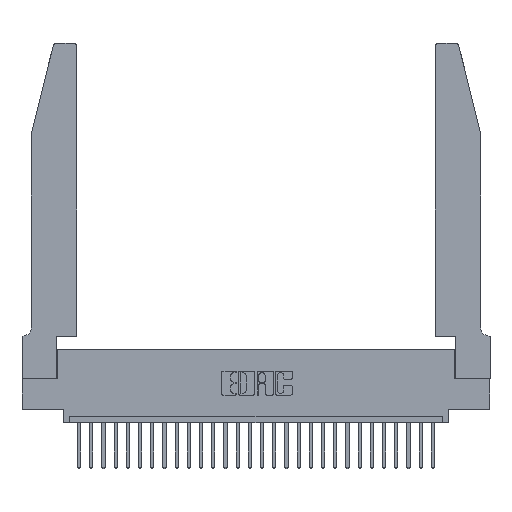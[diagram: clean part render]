
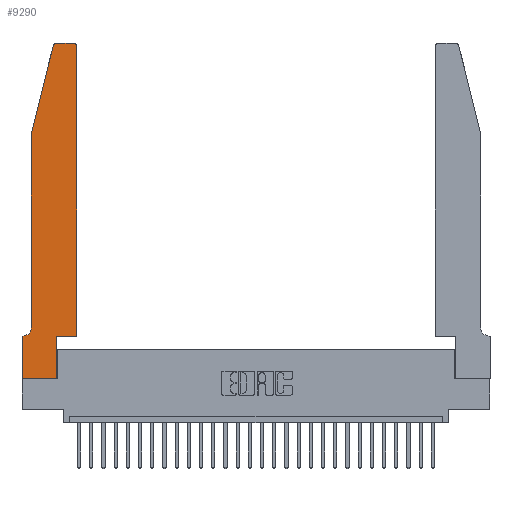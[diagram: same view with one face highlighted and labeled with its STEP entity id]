
A CAD part, top view. The second image highlights one B-rep face of the part: STEP entity #9290.
In plain terms, the highlighted planar face has unit normal (0, 0, 1).
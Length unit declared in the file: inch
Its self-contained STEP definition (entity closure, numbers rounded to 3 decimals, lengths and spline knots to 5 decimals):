
#33 = VERTEX_POINT ( 'NONE', #4199 ) ;
#1067 = VERTEX_POINT ( 'NONE', #9888 ) ;
#1126 = CARTESIAN_POINT ( 'NONE',  ( 0.4505, 0.35, 0.37 ) ) ;
#1239 = CARTESIAN_POINT ( 'NONE',  ( 0.0755, 2., 0.37 ) ) ;
#1990 = EDGE_CURVE ( 'NONE', #8995, #33, #26808, .T. ) ;
#2002 = VERTEX_POINT ( 'NONE', #19369 ) ;
#2419 = ORIENTED_EDGE ( 'NONE', *, *, #24990, .T. ) ;
#3208 = EDGE_CURVE ( 'NONE', #8972, #7296, #18453, .T. ) ;
#3397 = AXIS2_PLACEMENT_3D ( 'NONE', #26261, #28527, #10773 ) ;
#3469 = EDGE_CURVE ( 'NONE', #1067, #24277, #12813, .T. ) ;
#3487 = CARTESIAN_POINT ( 'NONE',  ( 0.25487, 2.72718, 0.37 ) ) ;
#3885 = LINE ( 'NONE', #25903, #18589 ) ;
#3973 = LINE ( 'NONE', #25952, #18340 ) ;
#4199 = CARTESIAN_POINT ( 'NONE',  ( 0.4205, 2.75, 0.37 ) ) ;
#4271 = ORIENTED_EDGE ( 'NONE', *, *, #23421, .T. ) ;
#4342 = CARTESIAN_POINT ( 'NONE',  ( 0.284, 2.75, 0.37 ) ) ;
#4543 = ORIENTED_EDGE ( 'NONE', *, *, #11317, .T. ) ;
#4917 = EDGE_CURVE ( 'NONE', #33, #8972, #3973, .T. ) ;
#5338 = VECTOR ( 'NONE', #28657, 39.37008 ) ;
#5374 = DIRECTION ( 'NONE',  ( 1., 0., 0. ) ) ;
#6930 = CARTESIAN_POINT ( 'NONE',  ( 0.0755, 2., 0.37 ) ) ;
#7296 = VERTEX_POINT ( 'NONE', #3487 ) ;
#7378 = VECTOR ( 'NONE', #21597, 39.37008 ) ;
#7699 = DIRECTION ( 'NONE',  ( 0., -1., 0. ) ) ;
#8670 = AXIS2_PLACEMENT_3D ( 'NONE', #24192, #21921, #15005 ) ;
#8813 = DIRECTION ( 'NONE',  ( -1., 0., 0. ) ) ;
#8833 = ORIENTED_EDGE ( 'NONE', *, *, #3208, .T. ) ;
#8972 = VERTEX_POINT ( 'NONE', #4342 ) ;
#8995 = VERTEX_POINT ( 'NONE', #29036 ) ;
#9290 = ADVANCED_FACE ( 'NONE', ( #16309 ), #11573, .T. ) ;
#9346 = LINE ( 'NONE', #27927, #24161 ) ;
#9732 = ORIENTED_EDGE ( 'NONE', *, *, #11077, .T. ) ;
#9769 = CARTESIAN_POINT ( 'NONE',  ( 0., 0., 0.37 ) ) ;
#9888 = CARTESIAN_POINT ( 'NONE',  ( 0.2865, 0.35, 0.37 ) ) ;
#10009 = EDGE_LOOP ( 'NONE', ( #20983, #8833, #2419, #11010, #25842, #27282, #9732, #4271, #25207, #10694, #4543, #22345 ) ) ;
#10694 = ORIENTED_EDGE ( 'NONE', *, *, #3469, .T. ) ;
#10773 = DIRECTION ( 'NONE',  ( 1., 0., 0. ) ) ;
#11010 = ORIENTED_EDGE ( 'NONE', *, *, #20117, .T. ) ;
#11077 = EDGE_CURVE ( 'NONE', #20447, #13400, #21896, .T. ) ;
#11294 = VECTOR ( 'NONE', #7699, 39.37008 ) ;
#11317 = EDGE_CURVE ( 'NONE', #24277, #8995, #25748, .T. ) ;
#11573 = PLANE ( 'NONE',  #16643 ) ;
#11672 = DIRECTION ( 'NONE',  ( 0., 0., 1. ) ) ;
#11928 = EDGE_CURVE ( 'NONE', #13468, #1067, #25027, .T. ) ;
#12640 = DIRECTION ( 'NONE',  ( -0.239, -0.971, 0. ) ) ;
#12813 = LINE ( 'NONE', #15622, #26584 ) ;
#13247 = CARTESIAN_POINT ( 'NONE',  ( 0.2865, 0., 0.37 ) ) ;
#13400 = VERTEX_POINT ( 'NONE', #27372 ) ;
#13468 = VERTEX_POINT ( 'NONE', #13247 ) ;
#13855 = VERTEX_POINT ( 'NONE', #6930 ) ;
#14664 = CARTESIAN_POINT ( 'NONE',  ( 0.0055, 0.35, 0.37 ) ) ;
#15005 = DIRECTION ( 'NONE',  ( 1., 0., 0. ) ) ;
#15314 = EDGE_CURVE ( 'NONE', #2002, #24054, #16683, .T. ) ;
#15622 = CARTESIAN_POINT ( 'NONE',  ( 0.4505, 0.35, 0.37 ) ) ;
#15716 = DIRECTION ( 'NONE',  ( 1., 0., 0. ) ) ;
#16197 = EDGE_CURVE ( 'NONE', #24054, #20447, #25414, .T. ) ;
#16309 = FACE_OUTER_BOUND ( 'NONE', #10009, .T. ) ;
#16603 = DIRECTION ( 'NONE',  ( 0., 1., 0. ) ) ;
#16643 = AXIS2_PLACEMENT_3D ( 'NONE', #25199, #11672, #27349 ) ;
#16677 = DIRECTION ( 'NONE',  ( 0., -1., 0. ) ) ;
#16683 = CIRCLE ( 'NONE', #23227, 0.07 ) ;
#17084 = VECTOR ( 'NONE', #12640, 39.37008 ) ;
#17344 = CARTESIAN_POINT ( 'NONE',  ( 0.2865, 0.35, 0.37 ) ) ;
#17428 = LINE ( 'NONE', #1239, #17084 ) ;
#18340 = VECTOR ( 'NONE', #28215, 39.37008 ) ;
#18453 = CIRCLE ( 'NONE', #8670, 0.03 ) ;
#18589 = VECTOR ( 'NONE', #5374, 39.37008 ) ;
#19369 = CARTESIAN_POINT ( 'NONE',  ( 0.0755, 0.42, 0.37 ) ) ;
#19756 = VECTOR ( 'NONE', #16603, 39.37008 ) ;
#20117 = EDGE_CURVE ( 'NONE', #13855, #2002, #9346, .T. ) ;
#20447 = VERTEX_POINT ( 'NONE', #24568 ) ;
#20983 = ORIENTED_EDGE ( 'NONE', *, *, #4917, .T. ) ;
#21597 = DIRECTION ( 'NONE',  ( 0., 1., 0. ) ) ;
#21896 = LINE ( 'NONE', #9769, #11294 ) ;
#21921 = DIRECTION ( 'NONE',  ( 0., 0., 1. ) ) ;
#22345 = ORIENTED_EDGE ( 'NONE', *, *, #1990, .T. ) ;
#23227 = AXIS2_PLACEMENT_3D ( 'NONE', #25645, #25742, #8813 ) ;
#23421 = EDGE_CURVE ( 'NONE', #13400, #13468, #3885, .T. ) ;
#24054 = VERTEX_POINT ( 'NONE', #14664 ) ;
#24161 = VECTOR ( 'NONE', #16677, 39.37008 ) ;
#24192 = CARTESIAN_POINT ( 'NONE',  ( 0.284, 2.72, 0.37 ) ) ;
#24277 = VERTEX_POINT ( 'NONE', #1126 ) ;
#24436 = CARTESIAN_POINT ( 'NONE',  ( 0.0755, 0.35, 0.37 ) ) ;
#24568 = CARTESIAN_POINT ( 'NONE',  ( 0., 0.35, 0.37 ) ) ;
#24990 = EDGE_CURVE ( 'NONE', #7296, #13855, #17428, .T. ) ;
#25027 = LINE ( 'NONE', #17344, #7378 ) ;
#25199 = CARTESIAN_POINT ( 'NONE',  ( 0., 0.35, 0.37 ) ) ;
#25207 = ORIENTED_EDGE ( 'NONE', *, *, #11928, .T. ) ;
#25414 = LINE ( 'NONE', #24436, #5338 ) ;
#25645 = CARTESIAN_POINT ( 'NONE',  ( 0.0055, 0.42, 0.37 ) ) ;
#25742 = DIRECTION ( 'NONE',  ( 0., 0., -1. ) ) ;
#25748 = LINE ( 'NONE', #28050, #19756 ) ;
#25842 = ORIENTED_EDGE ( 'NONE', *, *, #15314, .T. ) ;
#25903 = CARTESIAN_POINT ( 'NONE',  ( 0., 0., 0.37 ) ) ;
#25952 = CARTESIAN_POINT ( 'NONE',  ( 0.2605, 2.75, 0.37 ) ) ;
#26261 = CARTESIAN_POINT ( 'NONE',  ( 0.4205, 2.72, 0.37 ) ) ;
#26584 = VECTOR ( 'NONE', #15716, 39.37008 ) ;
#26808 = CIRCLE ( 'NONE', #3397, 0.03 ) ;
#27282 = ORIENTED_EDGE ( 'NONE', *, *, #16197, .T. ) ;
#27349 = DIRECTION ( 'NONE',  ( 1., 0., 0. ) ) ;
#27372 = CARTESIAN_POINT ( 'NONE',  ( 0., 0., 0.37 ) ) ;
#27927 = CARTESIAN_POINT ( 'NONE',  ( 0.0755, 2., 0.37 ) ) ;
#28050 = CARTESIAN_POINT ( 'NONE',  ( 0.4505, 0.35, 0.37 ) ) ;
#28215 = DIRECTION ( 'NONE',  ( -1., 0., 0. ) ) ;
#28527 = DIRECTION ( 'NONE',  ( 0., 0., 1. ) ) ;
#28657 = DIRECTION ( 'NONE',  ( -1., 0., 0. ) ) ;
#29036 = CARTESIAN_POINT ( 'NONE',  ( 0.4505, 2.72, 0.37 ) ) ;
